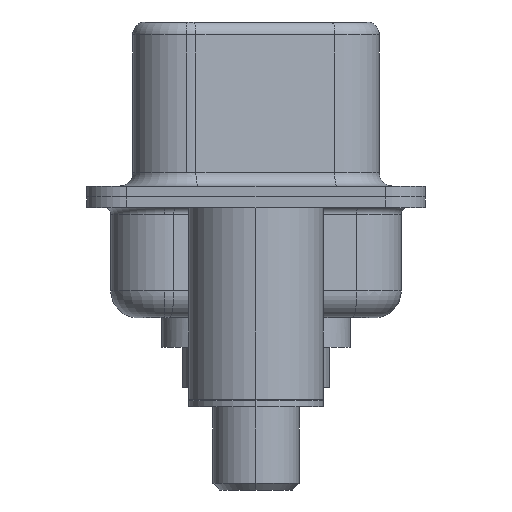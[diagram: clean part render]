
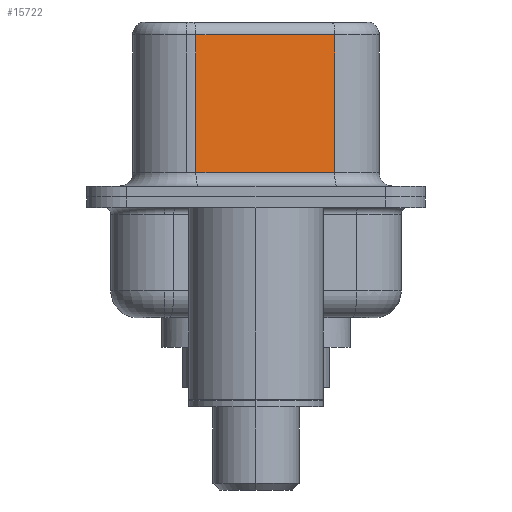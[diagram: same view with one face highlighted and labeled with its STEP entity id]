
A CAD part, left-side view. The second image highlights one B-rep face of the part: STEP entity #15722.
In plain terms, the highlighted planar face has unit normal (-0.985, -0.174, 0).
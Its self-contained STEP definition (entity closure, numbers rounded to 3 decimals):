
#695 = EDGE_CURVE ( 'NONE', #17756, #5586, #1000, .T. ) ;
#810 = LINE ( 'NONE', #12633, #15609 ) ;
#1000 = LINE ( 'NONE', #7102, #9066 ) ;
#1638 = DIRECTION ( 'NONE',  ( 0., 0., -1. ) ) ;
#1994 = VECTOR ( 'NONE', #18314, 1000. ) ;
#3068 = CARTESIAN_POINT ( 'NONE',  ( 4.585, -2.927, 6.52 ) ) ;
#4514 = DIRECTION ( 'NONE',  ( -0.174, 0.985, 0. ) ) ;
#4562 = CARTESIAN_POINT ( 'NONE',  ( 4.585, -2.927, 6.02 ) ) ;
#5214 = VECTOR ( 'NONE', #14841, 1000. ) ;
#5541 = EDGE_CURVE ( 'NONE', #5586, #5823, #16642, .T. ) ;
#5586 = VERTEX_POINT ( 'NONE', #9256 ) ;
#5823 = VERTEX_POINT ( 'NONE', #8512 ) ;
#6321 = ORIENTED_EDGE ( 'NONE', *, *, #5541, .T. ) ;
#6402 = PLANE ( 'NONE',  #15594 ) ;
#7102 = CARTESIAN_POINT ( 'NONE',  ( 3.675, 2.233, 6.52 ) ) ;
#8512 = CARTESIAN_POINT ( 'NONE',  ( 4.585, -2.927, 0.9 ) ) ;
#8760 = ORIENTED_EDGE ( 'NONE', *, *, #695, .T. ) ;
#8847 = CARTESIAN_POINT ( 'NONE',  ( 3.675, 2.233, 6.02 ) ) ;
#9066 = VECTOR ( 'NONE', #1638, 1000. ) ;
#9256 = CARTESIAN_POINT ( 'NONE',  ( 3.675, 2.233, 0.9 ) ) ;
#9655 = CARTESIAN_POINT ( 'NONE',  ( 4.585, -2.927, 6.02 ) ) ;
#11286 = EDGE_CURVE ( 'NONE', #18475, #5823, #810, .T. ) ;
#11936 = ORIENTED_EDGE ( 'NONE', *, *, #11286, .F. ) ;
#12633 = CARTESIAN_POINT ( 'NONE',  ( 4.585, -2.927, 6.52 ) ) ;
#13062 = DIRECTION ( 'NONE',  ( 0.985, 0.174, 0. ) ) ;
#13471 = FACE_OUTER_BOUND ( 'NONE', #16014, .T. ) ;
#14841 = DIRECTION ( 'NONE',  ( 0.174, -0.985, 0. ) ) ;
#14935 = CARTESIAN_POINT ( 'NONE',  ( 4.585, -2.927, 0.9 ) ) ;
#15594 = AXIS2_PLACEMENT_3D ( 'NONE', #3068, #13062, #4514 ) ;
#15609 = VECTOR ( 'NONE', #16986, 1000. ) ;
#15722 = ADVANCED_FACE ( 'NONE', ( #13471 ), #6402, .F. ) ;
#16014 = EDGE_LOOP ( 'NONE', ( #11936, #16556, #8760, #6321 ) ) ;
#16556 = ORIENTED_EDGE ( 'NONE', *, *, #17477, .T. ) ;
#16642 = LINE ( 'NONE', #14935, #5214 ) ;
#16805 = LINE ( 'NONE', #9655, #1994 ) ;
#16986 = DIRECTION ( 'NONE',  ( 0., 0., -1. ) ) ;
#17477 = EDGE_CURVE ( 'NONE', #18475, #17756, #16805, .T. ) ;
#17756 = VERTEX_POINT ( 'NONE', #8847 ) ;
#18314 = DIRECTION ( 'NONE',  ( -0.174, 0.985, 0. ) ) ;
#18475 = VERTEX_POINT ( 'NONE', #4562 ) ;
